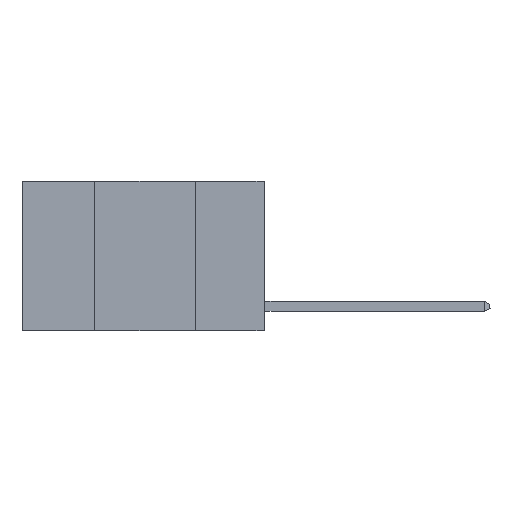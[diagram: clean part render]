
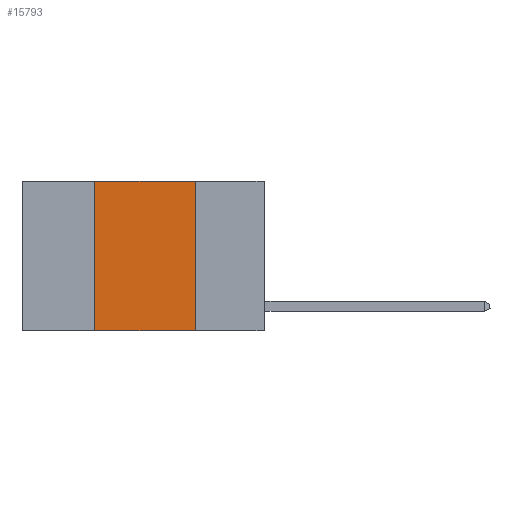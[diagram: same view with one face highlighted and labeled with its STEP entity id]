
A CAD part, left-side view. The second image highlights one B-rep face of the part: STEP entity #15793.
In plain terms, the highlighted planar face has unit normal (-1, 0, 0).
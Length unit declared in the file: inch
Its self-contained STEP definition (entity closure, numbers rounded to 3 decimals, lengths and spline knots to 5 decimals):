
#49 = DIRECTION ( 'NONE',  ( 0., 0., -1. ) ) ;
#1049 = CARTESIAN_POINT ( 'NONE',  ( 0., 0.42, -0.37 ) ) ;
#1256 = CARTESIAN_POINT ( 'NONE',  ( 0., 0.6, -0.37 ) ) ;
#1344 = DIRECTION ( 'NONE',  ( 0., -1., 0. ) ) ;
#1728 = VERTEX_POINT ( 'NONE', #15812 ) ;
#1887 = ORIENTED_EDGE ( 'NONE', *, *, #7882, .T. ) ;
#2278 = EDGE_LOOP ( 'NONE', ( #7513, #11541, #2783, #1887 ) ) ;
#2783 = ORIENTED_EDGE ( 'NONE', *, *, #14068, .F. ) ;
#3482 = CARTESIAN_POINT ( 'NONE',  ( 0., 0.6, 0. ) ) ;
#3584 = VECTOR ( 'NONE', #6901, 39.37008 ) ;
#4040 = VERTEX_POINT ( 'NONE', #1049 ) ;
#5442 = CARTESIAN_POINT ( 'NONE',  ( 0., 0.17, 0. ) ) ;
#6901 = DIRECTION ( 'NONE',  ( 0., 0., 1. ) ) ;
#7144 = VERTEX_POINT ( 'NONE', #11243 ) ;
#7489 = LINE ( 'NONE', #1256, #13617 ) ;
#7513 = ORIENTED_EDGE ( 'NONE', *, *, #14809, .F. ) ;
#7882 = EDGE_CURVE ( 'NONE', #4040, #7144, #7489, .T. ) ;
#7963 = EDGE_CURVE ( 'NONE', #1728, #12343, #14730, .T. ) ;
#8287 = CARTESIAN_POINT ( 'NONE',  ( 0., 0.42, 0. ) ) ;
#8483 = DIRECTION ( 'NONE',  ( 0., -1., 0. ) ) ;
#9927 = PLANE ( 'NONE',  #12257 ) ;
#11243 = CARTESIAN_POINT ( 'NONE',  ( 0., 0.17, -0.37 ) ) ;
#11298 = LINE ( 'NONE', #14918, #15661 ) ;
#11319 = DIRECTION ( 'NONE',  ( 0., 0., -1. ) ) ;
#11541 = ORIENTED_EDGE ( 'NONE', *, *, #7963, .F. ) ;
#12257 = AXIS2_PLACEMENT_3D ( 'NONE', #14940, #12465, #11319 ) ;
#12343 = VERTEX_POINT ( 'NONE', #5442 ) ;
#12465 = DIRECTION ( 'NONE',  ( 1., 0., 0. ) ) ;
#13617 = VECTOR ( 'NONE', #1344, 39.37008 ) ;
#14068 = EDGE_CURVE ( 'NONE', #4040, #1728, #14534, .T. ) ;
#14534 = LINE ( 'NONE', #8287, #3584 ) ;
#14701 = VECTOR ( 'NONE', #8483, 39.37008 ) ;
#14730 = LINE ( 'NONE', #3482, #14701 ) ;
#14809 = EDGE_CURVE ( 'NONE', #12343, #7144, #11298, .T. ) ;
#14918 = CARTESIAN_POINT ( 'NONE',  ( 0., 0.17, 0. ) ) ;
#14940 = CARTESIAN_POINT ( 'NONE',  ( 0., 0.6, 0. ) ) ;
#15661 = VECTOR ( 'NONE', #49, 39.37008 ) ;
#15793 = ADVANCED_FACE ( 'NONE', ( #16176 ), #9927, .F. ) ;
#15812 = CARTESIAN_POINT ( 'NONE',  ( 0., 0.42, 0. ) ) ;
#16176 = FACE_OUTER_BOUND ( 'NONE', #2278, .T. ) ;
